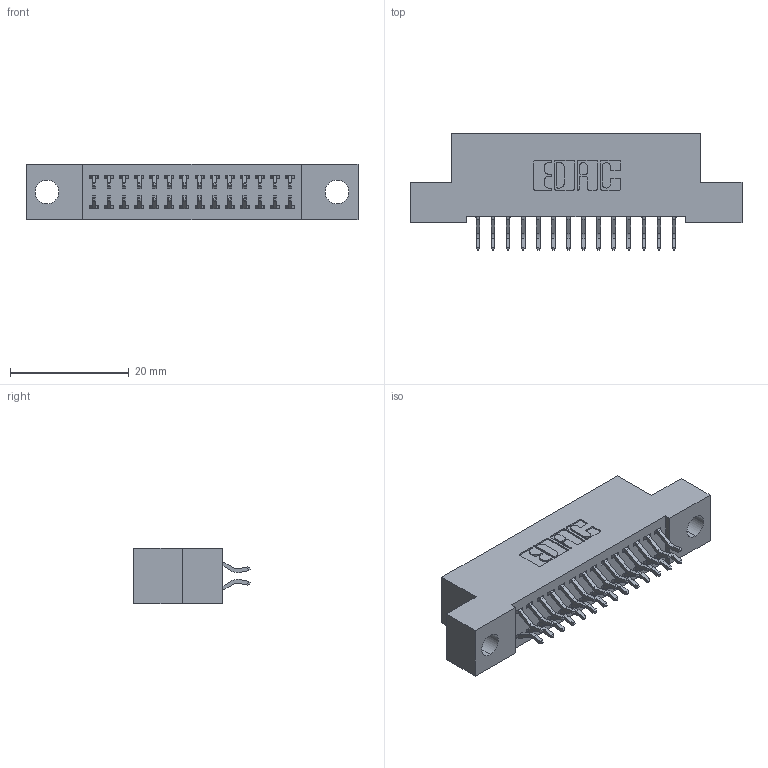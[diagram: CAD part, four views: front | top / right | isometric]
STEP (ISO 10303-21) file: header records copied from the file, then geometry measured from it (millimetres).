
FILE_DESCRIPTION (( 'STEP AP203' ), '1' );
FILE_NAME ('342-028-556-204.STEP', '2018-08-11T14:27:20', ( '' ), ( '' ), 'SwSTEP 2.0', 'SolidWorks 2016', '' );
FILE_SCHEMA (( 'CONFIG_CONTROL_DESIGN' ));
Length unit declared in the file: inch
Products named in the file (3): 342 Part_.156 TH; 345-292-001_556 Tail; 342-028-556-204
Assembly tree (29 placements, depth 2):
  342-028-556-204
    342 Part_.156 TH
    345-292-001_556 Tail  x28
Bounding box: 55.88 x 19.58 x 9.4 mm (x, y, z)
Volume: 4800.5 mm3; surface area: 6921.2 mm2
Topology: 29 solids, 29 shells, 1734 faces, 5143 edges, 3390 vertices
Faces by surface type: plane 1186, cylinder 548
Entity records: 12719 total; most frequent: CARTESIAN_POINT 2154, ORIENTED_EDGE 2078, DIRECTION 1879, EDGE_CURVE 1039, VECTOR 903, LINE 903, VERTEX_POINT 690, AXIS2_PLACEMENT_3D 488
